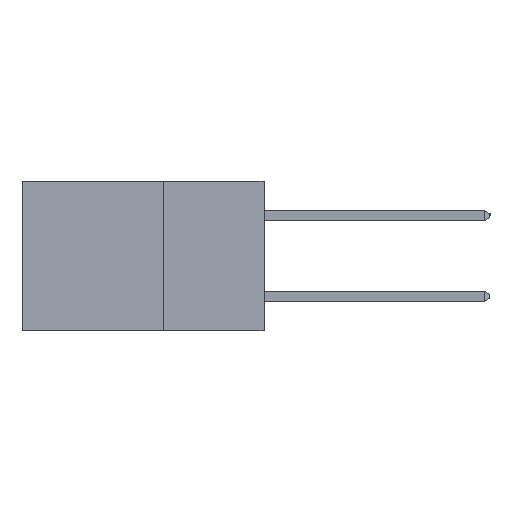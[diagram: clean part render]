
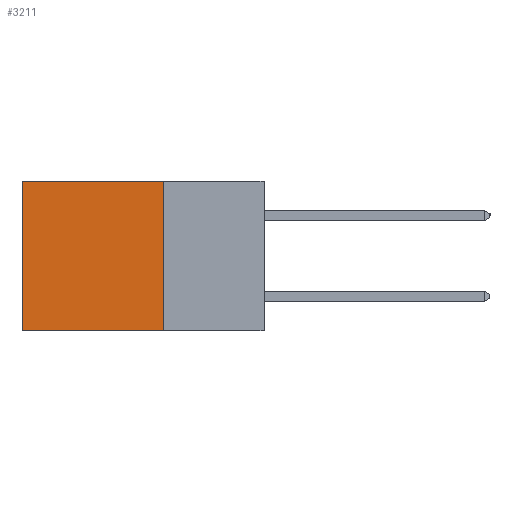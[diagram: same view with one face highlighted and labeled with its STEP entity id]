
A CAD part, left-side view. The second image highlights one B-rep face of the part: STEP entity #3211.
In plain terms, the highlighted planar face has unit normal (-1, 0, 0).
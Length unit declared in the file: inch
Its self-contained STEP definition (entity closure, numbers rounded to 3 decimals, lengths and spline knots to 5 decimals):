
#425 = EDGE_CURVE ( 'NONE', #8656, #17497, #5922, .T. ) ;
#1247 = DIRECTION ( 'NONE',  ( 0., 0., -1. ) ) ;
#1592 = DIRECTION ( 'NONE',  ( 0., 0., -1. ) ) ;
#1840 = VECTOR ( 'NONE', #2524, 39.37008 ) ;
#1856 = EDGE_CURVE ( 'NONE', #17497, #4338, #11291, .T. ) ;
#2524 = DIRECTION ( 'NONE',  ( 0., 1., 0. ) ) ;
#2699 = VECTOR ( 'NONE', #3223, 39.37008 ) ;
#3206 = ORIENTED_EDGE ( 'NONE', *, *, #425, .T. ) ;
#3211 = ADVANCED_FACE ( 'NONE', ( #15067 ), #7888, .F. ) ;
#3223 = DIRECTION ( 'NONE',  ( 0., 1., 0. ) ) ;
#3277 = DIRECTION ( 'NONE',  ( 0., 0., -1. ) ) ;
#3845 = CARTESIAN_POINT ( 'NONE',  ( 0.2615, 0.25, -0.37 ) ) ;
#4338 = VERTEX_POINT ( 'NONE', #12457 ) ;
#5717 = CARTESIAN_POINT ( 'NONE',  ( 0.2615, 0.25, 0. ) ) ;
#5922 = LINE ( 'NONE', #5717, #1840 ) ;
#6272 = VECTOR ( 'NONE', #1247, 39.37008 ) ;
#7427 = CARTESIAN_POINT ( 'NONE',  ( 0.2615, 0.25, -0.37 ) ) ;
#7802 = AXIS2_PLACEMENT_3D ( 'NONE', #14234, #9246, #3277 ) ;
#7888 = PLANE ( 'NONE',  #7802 ) ;
#8656 = VERTEX_POINT ( 'NONE', #8934 ) ;
#8934 = CARTESIAN_POINT ( 'NONE',  ( 0.2615, 0.25, 0. ) ) ;
#8950 = CARTESIAN_POINT ( 'NONE',  ( 0.2615, 0.6, 0. ) ) ;
#9246 = DIRECTION ( 'NONE',  ( 1., 0., 0. ) ) ;
#9386 = VECTOR ( 'NONE', #1592, 39.37008 ) ;
#9570 = ORIENTED_EDGE ( 'NONE', *, *, #15462, .F. ) ;
#11291 = LINE ( 'NONE', #12659, #9386 ) ;
#12102 = ORIENTED_EDGE ( 'NONE', *, *, #14418, .F. ) ;
#12457 = CARTESIAN_POINT ( 'NONE',  ( 0.2615, 0.6, -0.37 ) ) ;
#12482 = VERTEX_POINT ( 'NONE', #3845 ) ;
#12659 = CARTESIAN_POINT ( 'NONE',  ( 0.2615, 0.6, -0.37 ) ) ;
#14234 = CARTESIAN_POINT ( 'NONE',  ( 0.2615, 0.25, -0.37 ) ) ;
#14418 = EDGE_CURVE ( 'NONE', #8656, #12482, #18799, .T. ) ;
#15067 = FACE_OUTER_BOUND ( 'NONE', #15711, .T. ) ;
#15319 = LINE ( 'NONE', #7427, #2699 ) ;
#15426 = CARTESIAN_POINT ( 'NONE',  ( 0.2615, 0.25, -0.37 ) ) ;
#15462 = EDGE_CURVE ( 'NONE', #12482, #4338, #15319, .T. ) ;
#15711 = EDGE_LOOP ( 'NONE', ( #20354, #9570, #12102, #3206 ) ) ;
#17497 = VERTEX_POINT ( 'NONE', #8950 ) ;
#18799 = LINE ( 'NONE', #15426, #6272 ) ;
#20354 = ORIENTED_EDGE ( 'NONE', *, *, #1856, .T. ) ;
